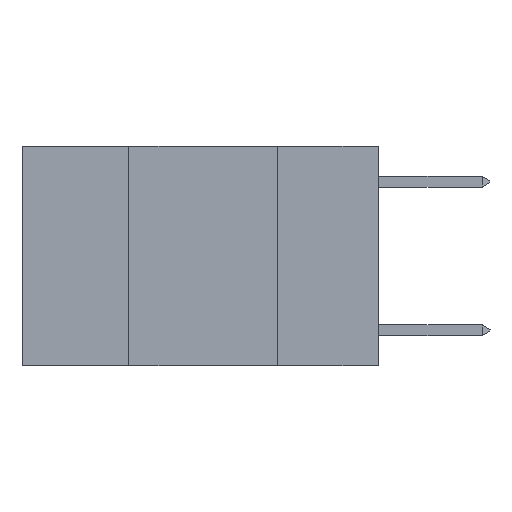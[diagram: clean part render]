
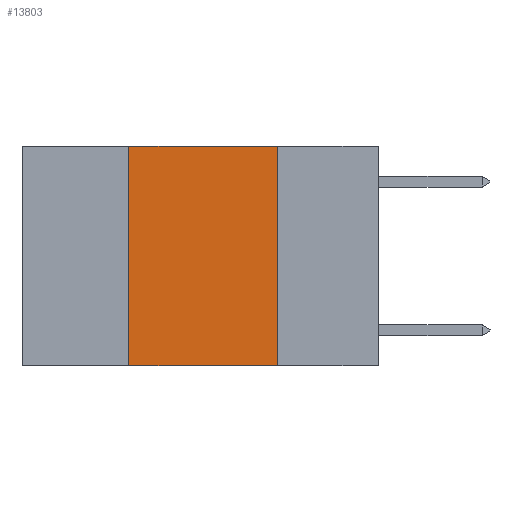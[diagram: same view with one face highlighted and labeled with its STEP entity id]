
A CAD part, left-side view. The second image highlights one B-rep face of the part: STEP entity #13803.
In plain terms, the highlighted planar face has unit normal (-1, 0, 0).
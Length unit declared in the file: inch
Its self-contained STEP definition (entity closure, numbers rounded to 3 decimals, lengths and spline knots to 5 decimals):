
#578 = CARTESIAN_POINT ( 'NONE',  ( 0., 0.42, 0. ) ) ;
#709 = LINE ( 'NONE', #578, #12711 ) ;
#2010 = VECTOR ( 'NONE', #7832, 39.37008 ) ;
#3018 = DIRECTION ( 'NONE',  ( 0., 0., 1. ) ) ;
#4324 = VECTOR ( 'NONE', #9958, 39.37008 ) ;
#5613 = LINE ( 'NONE', #25564, #17387 ) ;
#5635 = CARTESIAN_POINT ( 'NONE',  ( 0., 0.6, 0. ) ) ;
#7426 = CARTESIAN_POINT ( 'NONE',  ( 0., 0.17, -0.37 ) ) ;
#7832 = DIRECTION ( 'NONE',  ( 0., -1., 0. ) ) ;
#8294 = FACE_OUTER_BOUND ( 'NONE', #15036, .T. ) ;
#9234 = LINE ( 'NONE', #26199, #4324 ) ;
#9958 = DIRECTION ( 'NONE',  ( 0., 0., -1. ) ) ;
#10411 = DIRECTION ( 'NONE',  ( 0., 0., -1. ) ) ;
#10470 = VERTEX_POINT ( 'NONE', #13754 ) ;
#11606 = CARTESIAN_POINT ( 'NONE',  ( 0., 0.42, -0.37 ) ) ;
#12183 = VERTEX_POINT ( 'NONE', #11606 ) ;
#12711 = VECTOR ( 'NONE', #3018, 39.37008 ) ;
#13754 = CARTESIAN_POINT ( 'NONE',  ( 0., 0.42, 0. ) ) ;
#13803 = ADVANCED_FACE ( 'NONE', ( #8294 ), #19644, .F. ) ;
#14014 = LINE ( 'NONE', #28745, #2010 ) ;
#14045 = EDGE_CURVE ( 'NONE', #12183, #10470, #709, .T. ) ;
#15036 = EDGE_LOOP ( 'NONE', ( #29723, #18121, #27145, #29030 ) ) ;
#17387 = VECTOR ( 'NONE', #27889, 39.37008 ) ;
#17478 = AXIS2_PLACEMENT_3D ( 'NONE', #5635, #24283, #10411 ) ;
#18121 = ORIENTED_EDGE ( 'NONE', *, *, #21134, .F. ) ;
#19644 = PLANE ( 'NONE',  #17478 ) ;
#21134 = EDGE_CURVE ( 'NONE', #10470, #27447, #5613, .T. ) ;
#22070 = CARTESIAN_POINT ( 'NONE',  ( 0., 0.17, 0. ) ) ;
#24283 = DIRECTION ( 'NONE',  ( 1., 0., 0. ) ) ;
#25564 = CARTESIAN_POINT ( 'NONE',  ( 0., 0.6, 0. ) ) ;
#26199 = CARTESIAN_POINT ( 'NONE',  ( 0., 0.17, 0. ) ) ;
#26616 = EDGE_CURVE ( 'NONE', #27447, #27266, #9234, .T. ) ;
#27145 = ORIENTED_EDGE ( 'NONE', *, *, #14045, .F. ) ;
#27266 = VERTEX_POINT ( 'NONE', #7426 ) ;
#27351 = EDGE_CURVE ( 'NONE', #12183, #27266, #14014, .T. ) ;
#27447 = VERTEX_POINT ( 'NONE', #22070 ) ;
#27889 = DIRECTION ( 'NONE',  ( 0., -1., 0. ) ) ;
#28745 = CARTESIAN_POINT ( 'NONE',  ( 0., 0.6, -0.37 ) ) ;
#29030 = ORIENTED_EDGE ( 'NONE', *, *, #27351, .T. ) ;
#29723 = ORIENTED_EDGE ( 'NONE', *, *, #26616, .F. ) ;
